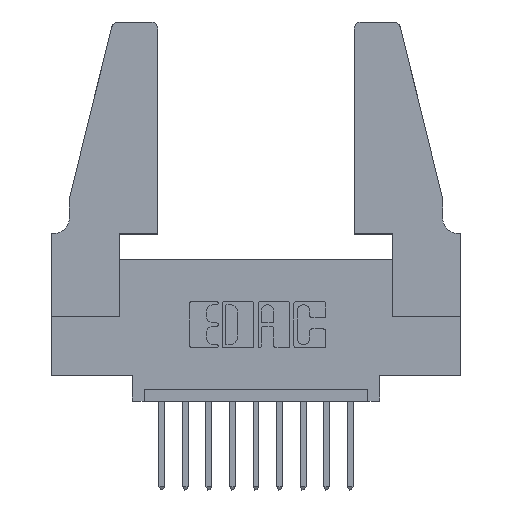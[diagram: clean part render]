
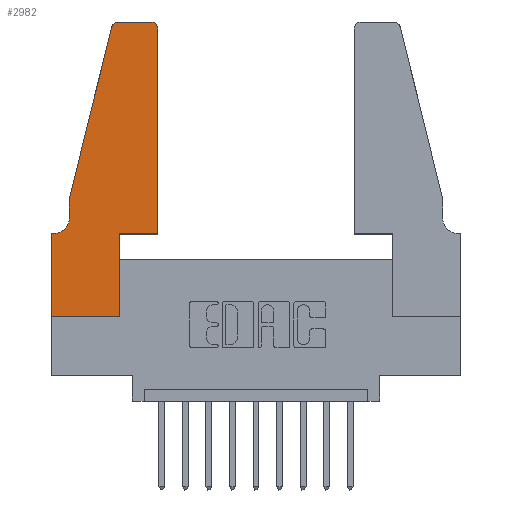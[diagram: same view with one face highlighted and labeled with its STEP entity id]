
A CAD part, top view. The second image highlights one B-rep face of the part: STEP entity #2982.
In plain terms, the highlighted planar face has unit normal (0, 0, 1).
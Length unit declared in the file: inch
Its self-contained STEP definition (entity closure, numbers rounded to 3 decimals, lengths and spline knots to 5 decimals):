
#2 = DIRECTION ( 'NONE',  ( 1., 0., 0. ) ) ;
#166 = DIRECTION ( 'NONE',  ( -0.239, -0.971, 0. ) ) ;
#217 = ORIENTED_EDGE ( 'NONE', *, *, #5014, .T. ) ;
#337 = DIRECTION ( 'NONE',  ( 0., -1., 0. ) ) ;
#479 = LINE ( 'NONE', #12693, #5033 ) ;
#1032 = CARTESIAN_POINT ( 'NONE',  ( 0.0055, 0.42, 0.37 ) ) ;
#1115 = VECTOR ( 'NONE', #5518, 39.37008 ) ;
#1126 = DIRECTION ( 'NONE',  ( 0., 0., -1. ) ) ;
#1286 = ORIENTED_EDGE ( 'NONE', *, *, #10876, .T. ) ;
#1458 = ORIENTED_EDGE ( 'NONE', *, *, #7105, .T. ) ;
#1510 = VERTEX_POINT ( 'NONE', #10666 ) ;
#1520 = CARTESIAN_POINT ( 'NONE',  ( 0.0755, 0.35, 0.37 ) ) ;
#1524 = ORIENTED_EDGE ( 'NONE', *, *, #6571, .T. ) ;
#1540 = ORIENTED_EDGE ( 'NONE', *, *, #13127, .T. ) ;
#1603 = CARTESIAN_POINT ( 'NONE',  ( 0.4205, 1.22, 0.37 ) ) ;
#1933 = VECTOR ( 'NONE', #11378, 39.37008 ) ;
#2074 = PLANE ( 'NONE',  #7529 ) ;
#2083 = DIRECTION ( 'NONE',  ( -1., 0., 0. ) ) ;
#2120 = VERTEX_POINT ( 'NONE', #9721 ) ;
#2294 = LINE ( 'NONE', #5796, #13105 ) ;
#2661 = EDGE_LOOP ( 'NONE', ( #1524, #12614, #1458, #11560, #1286, #6451, #13254, #217, #1540, #10090, #6128, #5647 ) ) ;
#2704 = DIRECTION ( 'NONE',  ( -1., 0., 0. ) ) ;
#2859 = VERTEX_POINT ( 'NONE', #4865 ) ;
#2938 = DIRECTION ( 'NONE',  ( 0., 1., 0. ) ) ;
#2982 = ADVANCED_FACE ( 'NONE', ( #7786 ), #2074, .T. ) ;
#3643 = LINE ( 'NONE', #11320, #13293 ) ;
#3712 = VERTEX_POINT ( 'NONE', #11737 ) ;
#3970 = CARTESIAN_POINT ( 'NONE',  ( 0., 0.35, 0.37 ) ) ;
#3996 = EDGE_CURVE ( 'NONE', #12258, #5404, #5942, .T. ) ;
#4046 = EDGE_CURVE ( 'NONE', #6676, #7395, #13161, .T. ) ;
#4707 = DIRECTION ( 'NONE',  ( 0., -1., 0. ) ) ;
#4755 = CARTESIAN_POINT ( 'NONE',  ( 0., 0., 0.37 ) ) ;
#4785 = CARTESIAN_POINT ( 'NONE',  ( 0., 0., 0.37 ) ) ;
#4856 = VERTEX_POINT ( 'NONE', #7875 ) ;
#4865 = CARTESIAN_POINT ( 'NONE',  ( 0.0755, 0.5, 0.37 ) ) ;
#5014 = EDGE_CURVE ( 'NONE', #5404, #2120, #3643, .T. ) ;
#5026 = LINE ( 'NONE', #11802, #1115 ) ;
#5033 = VECTOR ( 'NONE', #166, 39.37008 ) ;
#5162 = CARTESIAN_POINT ( 'NONE',  ( 0.25487, 1.22718, 0.37 ) ) ;
#5254 = CARTESIAN_POINT ( 'NONE',  ( 0.284, 1.22, 0.37 ) ) ;
#5404 = VERTEX_POINT ( 'NONE', #4785 ) ;
#5518 = DIRECTION ( 'NONE',  ( 1., 0., 0. ) ) ;
#5589 = DIRECTION ( 'NONE',  ( -1., 0., 0. ) ) ;
#5647 = ORIENTED_EDGE ( 'NONE', *, *, #4046, .T. ) ;
#5796 = CARTESIAN_POINT ( 'NONE',  ( 0.2605, 1.25, 0.37 ) ) ;
#5942 = LINE ( 'NONE', #4755, #11202 ) ;
#6128 = ORIENTED_EDGE ( 'NONE', *, *, #7852, .T. ) ;
#6138 = CIRCLE ( 'NONE', #10075, 0.07 ) ;
#6202 = VECTOR ( 'NONE', #337, 39.37008 ) ;
#6300 = DIRECTION ( 'NONE',  ( 0., 0., 1. ) ) ;
#6451 = ORIENTED_EDGE ( 'NONE', *, *, #7490, .T. ) ;
#6513 = EDGE_CURVE ( 'NONE', #2859, #3712, #8975, .T. ) ;
#6571 = EDGE_CURVE ( 'NONE', #7395, #11371, #2294, .T. ) ;
#6595 = LINE ( 'NONE', #8813, #7235 ) ;
#6676 = VERTEX_POINT ( 'NONE', #9867 ) ;
#7105 = EDGE_CURVE ( 'NONE', #7330, #2859, #479, .T. ) ;
#7235 = VECTOR ( 'NONE', #2938, 39.37008 ) ;
#7307 = DIRECTION ( 'NONE',  ( 0., 0., 1. ) ) ;
#7330 = VERTEX_POINT ( 'NONE', #5162 ) ;
#7395 = VERTEX_POINT ( 'NONE', #12679 ) ;
#7476 = CARTESIAN_POINT ( 'NONE',  ( 0.0055, 0.35, 0.37 ) ) ;
#7490 = EDGE_CURVE ( 'NONE', #9384, #12258, #11125, .T. ) ;
#7526 = CARTESIAN_POINT ( 'NONE',  ( 0.0755, 0.5, 0.37 ) ) ;
#7529 = AXIS2_PLACEMENT_3D ( 'NONE', #9355, #7307, #8405 ) ;
#7786 = FACE_OUTER_BOUND ( 'NONE', #2661, .T. ) ;
#7852 = EDGE_CURVE ( 'NONE', #4856, #6676, #12273, .T. ) ;
#7875 = CARTESIAN_POINT ( 'NONE',  ( 0.4505, 0.35, 0.37 ) ) ;
#8146 = AXIS2_PLACEMENT_3D ( 'NONE', #1603, #8982, #10038 ) ;
#8405 = DIRECTION ( 'NONE',  ( 1., 0., 0. ) ) ;
#8808 = CIRCLE ( 'NONE', #12546, 0.03 ) ;
#8813 = CARTESIAN_POINT ( 'NONE',  ( 0.2865, 0.35, 0.37 ) ) ;
#8975 = LINE ( 'NONE', #7526, #6202 ) ;
#8982 = DIRECTION ( 'NONE',  ( 0., 0., 1. ) ) ;
#9202 = EDGE_CURVE ( 'NONE', #11371, #7330, #8808, .T. ) ;
#9355 = CARTESIAN_POINT ( 'NONE',  ( 0., 0.35, 0.37 ) ) ;
#9384 = VERTEX_POINT ( 'NONE', #7476 ) ;
#9721 = CARTESIAN_POINT ( 'NONE',  ( 0.2865, 0., 0.37 ) ) ;
#9735 = EDGE_CURVE ( 'NONE', #1510, #4856, #5026, .T. ) ;
#9867 = CARTESIAN_POINT ( 'NONE',  ( 0.4505, 1.22, 0.37 ) ) ;
#10038 = DIRECTION ( 'NONE',  ( 1., 0., 0. ) ) ;
#10075 = AXIS2_PLACEMENT_3D ( 'NONE', #1032, #1126, #2083 ) ;
#10090 = ORIENTED_EDGE ( 'NONE', *, *, #9735, .T. ) ;
#10099 = VECTOR ( 'NONE', #5589, 39.37008 ) ;
#10403 = DIRECTION ( 'NONE',  ( 1., 0., 0. ) ) ;
#10412 = CARTESIAN_POINT ( 'NONE',  ( 0.4505, 0.35, 0.37 ) ) ;
#10666 = CARTESIAN_POINT ( 'NONE',  ( 0.2865, 0.35, 0.37 ) ) ;
#10876 = EDGE_CURVE ( 'NONE', #3712, #9384, #6138, .T. ) ;
#11125 = LINE ( 'NONE', #1520, #10099 ) ;
#11202 = VECTOR ( 'NONE', #4707, 39.37008 ) ;
#11320 = CARTESIAN_POINT ( 'NONE',  ( 0., 0., 0.37 ) ) ;
#11371 = VERTEX_POINT ( 'NONE', #11442 ) ;
#11378 = DIRECTION ( 'NONE',  ( 0., 1., 0. ) ) ;
#11442 = CARTESIAN_POINT ( 'NONE',  ( 0.284, 1.25, 0.37 ) ) ;
#11560 = ORIENTED_EDGE ( 'NONE', *, *, #6513, .T. ) ;
#11737 = CARTESIAN_POINT ( 'NONE',  ( 0.0755, 0.42, 0.37 ) ) ;
#11802 = CARTESIAN_POINT ( 'NONE',  ( 0.4505, 0.35, 0.37 ) ) ;
#12258 = VERTEX_POINT ( 'NONE', #3970 ) ;
#12273 = LINE ( 'NONE', #10412, #1933 ) ;
#12546 = AXIS2_PLACEMENT_3D ( 'NONE', #5254, #6300, #2 ) ;
#12614 = ORIENTED_EDGE ( 'NONE', *, *, #9202, .T. ) ;
#12679 = CARTESIAN_POINT ( 'NONE',  ( 0.4205, 1.25, 0.37 ) ) ;
#12693 = CARTESIAN_POINT ( 'NONE',  ( 0.0755, 0.5, 0.37 ) ) ;
#13105 = VECTOR ( 'NONE', #2704, 39.37008 ) ;
#13127 = EDGE_CURVE ( 'NONE', #2120, #1510, #6595, .T. ) ;
#13161 = CIRCLE ( 'NONE', #8146, 0.03 ) ;
#13254 = ORIENTED_EDGE ( 'NONE', *, *, #3996, .T. ) ;
#13293 = VECTOR ( 'NONE', #10403, 39.37008 ) ;
